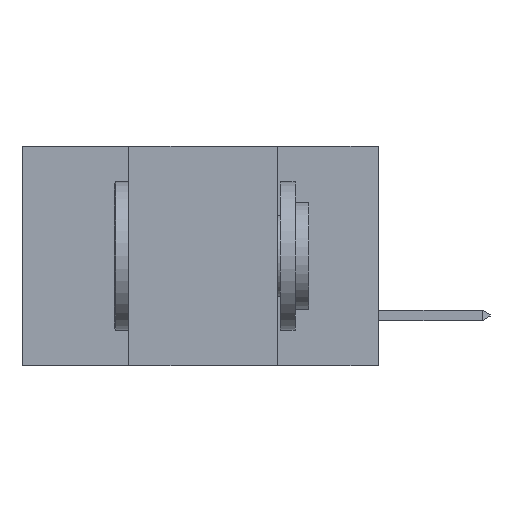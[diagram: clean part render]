
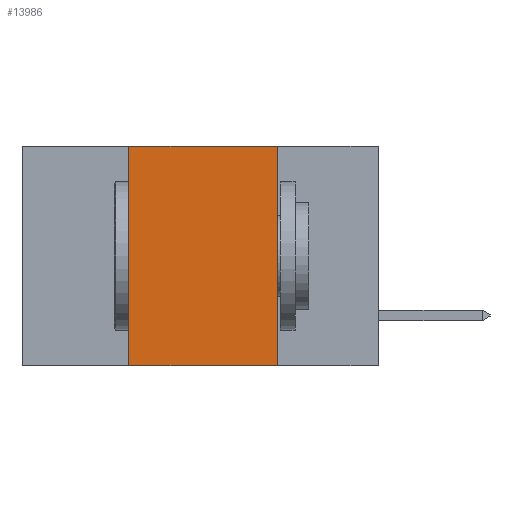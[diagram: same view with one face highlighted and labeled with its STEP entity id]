
A CAD part, left-side view. The second image highlights one B-rep face of the part: STEP entity #13986.
In plain terms, the highlighted planar face has unit normal (-1, 0, 0).
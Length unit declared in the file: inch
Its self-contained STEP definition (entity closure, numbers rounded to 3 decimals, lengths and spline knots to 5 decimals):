
#644 = EDGE_CURVE ( 'NONE', #2847, #11213, #13031, .T. ) ;
#1440 = ORIENTED_EDGE ( 'NONE', *, *, #644, .F. ) ;
#2586 = ORIENTED_EDGE ( 'NONE', *, *, #13895, .F. ) ;
#2752 = CARTESIAN_POINT ( 'NONE',  ( 0., 0.42, 0. ) ) ;
#2847 = VERTEX_POINT ( 'NONE', #14099 ) ;
#2959 = DIRECTION ( 'NONE',  ( 0., 0., -1. ) ) ;
#2978 = ORIENTED_EDGE ( 'NONE', *, *, #10775, .T. ) ;
#3258 = LINE ( 'NONE', #4016, #15932 ) ;
#3330 = VECTOR ( 'NONE', #12410, 39.37008 ) ;
#4016 = CARTESIAN_POINT ( 'NONE',  ( 0., 0.6, 0. ) ) ;
#4079 = CARTESIAN_POINT ( 'NONE',  ( 0., 0.42, -0.37 ) ) ;
#4589 = EDGE_LOOP ( 'NONE', ( #1440, #11640, #2586, #2978 ) ) ;
#5426 = PLANE ( 'NONE',  #12056 ) ;
#5594 = CARTESIAN_POINT ( 'NONE',  ( 0., 0.17, -0.37 ) ) ;
#6307 = CARTESIAN_POINT ( 'NONE',  ( 0., 0.6, -0.37 ) ) ;
#6460 = CARTESIAN_POINT ( 'NONE',  ( 0., 0.17, -0.37 ) ) ;
#7829 = DIRECTION ( 'NONE',  ( 0., 0., -1. ) ) ;
#8918 = DIRECTION ( 'NONE',  ( 0., -1., 0. ) ) ;
#9721 = VECTOR ( 'NONE', #7829, 39.37008 ) ;
#10335 = DIRECTION ( 'NONE',  ( 1., 0., 0. ) ) ;
#10561 = EDGE_CURVE ( 'NONE', #13870, #2847, #3258, .T. ) ;
#10775 = EDGE_CURVE ( 'NONE', #14069, #11213, #13183, .T. ) ;
#11213 = VERTEX_POINT ( 'NONE', #6460 ) ;
#11640 = ORIENTED_EDGE ( 'NONE', *, *, #10561, .F. ) ;
#11831 = VECTOR ( 'NONE', #12676, 39.37008 ) ;
#12056 = AXIS2_PLACEMENT_3D ( 'NONE', #15239, #10335, #2959 ) ;
#12410 = DIRECTION ( 'NONE',  ( 0., -1., 0. ) ) ;
#12676 = DIRECTION ( 'NONE',  ( 0., 0., 1. ) ) ;
#13011 = CARTESIAN_POINT ( 'NONE',  ( 0., 0.42, -0.37 ) ) ;
#13031 = LINE ( 'NONE', #5594, #9721 ) ;
#13183 = LINE ( 'NONE', #6307, #3330 ) ;
#13210 = FACE_OUTER_BOUND ( 'NONE', #4589, .T. ) ;
#13870 = VERTEX_POINT ( 'NONE', #2752 ) ;
#13895 = EDGE_CURVE ( 'NONE', #14069, #13870, #14358, .T. ) ;
#13986 = ADVANCED_FACE ( 'NONE', ( #13210 ), #5426, .F. ) ;
#14069 = VERTEX_POINT ( 'NONE', #13011 ) ;
#14099 = CARTESIAN_POINT ( 'NONE',  ( 0., 0.17, 0. ) ) ;
#14358 = LINE ( 'NONE', #4079, #11831 ) ;
#15239 = CARTESIAN_POINT ( 'NONE',  ( 0., 0.6, 0. ) ) ;
#15932 = VECTOR ( 'NONE', #8918, 39.37008 ) ;
